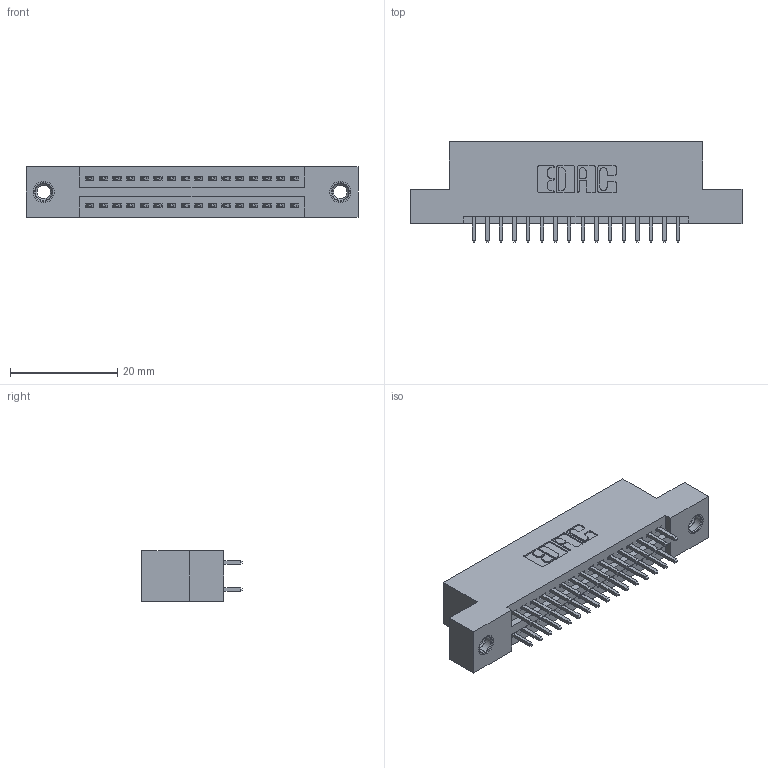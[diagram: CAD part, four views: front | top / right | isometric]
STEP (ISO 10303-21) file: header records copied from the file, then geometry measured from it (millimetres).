
FILE_DESCRIPTION (( 'STEP AP203' ), '1' );
FILE_NAME ('395-032-521-207.STEP', '2018-11-12T18:12:03', ( '' ), ( '' ), 'SwSTEP 2.0', 'SolidWorks 2016', '' );
FILE_SCHEMA (( 'CONFIG_CONTROL_DESIGN' ));
Length unit declared in the file: inch
Products named in the file (4): 345 Part_Flush Mounting Lugs - 0.156 Dia-TI; 395-032-521-207; 345-250-001_345-250-005-103; 345-292-001_345-293-121
Assembly tree (35 placements, depth 2):
  395-032-521-207
    345 Part_Flush Mounting Lugs - 0.156 Dia-TI
    345-292-001_345-293-121  x32
    345-250-001_345-250-005-103  x2
Bounding box: 61.85 x 18.72 x 9.4 mm (x, y, z)
Volume: 5740.2 mm3; surface area: 7924.2 mm2
Topology: 35 solids, 35 shells, 1786 faces, 5245 edges, 3446 vertices
Faces by surface type: plane 1168, cylinder 602, cone 12, torus 4
Entity records: 17258 total; most frequent: CARTESIAN_POINT 2899, ORIENTED_EDGE 2826, DIRECTION 2615, EDGE_CURVE 1413, LINE 1197, VECTOR 1197, VERTEX_POINT 936, AXIS2_PLACEMENT_3D 709
